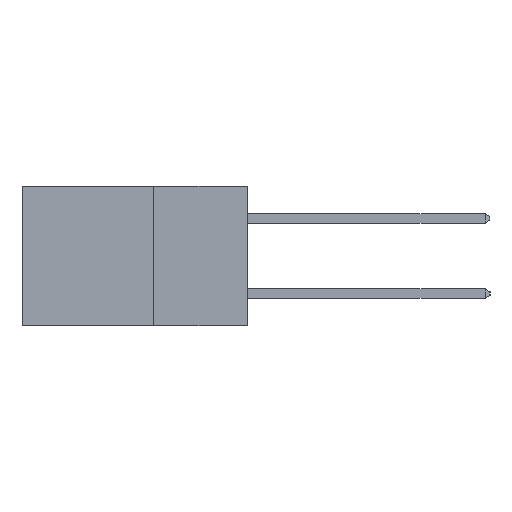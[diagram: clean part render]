
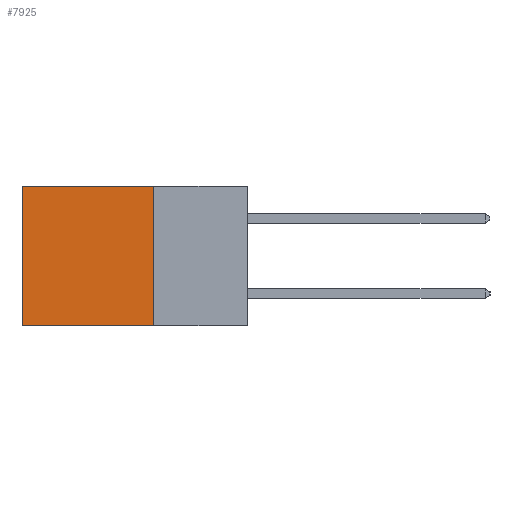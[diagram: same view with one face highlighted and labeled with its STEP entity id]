
A CAD part, left-side view. The second image highlights one B-rep face of the part: STEP entity #7925.
In plain terms, the highlighted planar face has unit normal (-1, 0, 0).
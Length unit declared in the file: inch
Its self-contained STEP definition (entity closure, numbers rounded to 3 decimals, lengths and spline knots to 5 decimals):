
#203 = LINE ( 'NONE', #7552, #11083 ) ;
#416 = DIRECTION ( 'NONE',  ( 0., 0., -1. ) ) ;
#539 = CARTESIAN_POINT ( 'NONE',  ( 0.2615, 0.6, -0.37 ) ) ;
#847 = CARTESIAN_POINT ( 'NONE',  ( 0.2615, 0.6, 0. ) ) ;
#979 = CARTESIAN_POINT ( 'NONE',  ( 0.2615, 0.25, -0.37 ) ) ;
#1391 = ORIENTED_EDGE ( 'NONE', *, *, #9194, .F. ) ;
#1603 = DIRECTION ( 'NONE',  ( 0., 1., 0. ) ) ;
#1889 = DIRECTION ( 'NONE',  ( 1., 0., 0. ) ) ;
#2540 = EDGE_CURVE ( 'NONE', #7242, #8028, #10541, .T. ) ;
#2684 = VECTOR ( 'NONE', #7913, 39.37008 ) ;
#3833 = PLANE ( 'NONE',  #10308 ) ;
#5373 = CARTESIAN_POINT ( 'NONE',  ( 0.2615, 0.25, -0.37 ) ) ;
#5421 = CARTESIAN_POINT ( 'NONE',  ( 0.2615, 0.25, -0.37 ) ) ;
#5601 = VERTEX_POINT ( 'NONE', #5373 ) ;
#5627 = EDGE_CURVE ( 'NONE', #7146, #5601, #10991, .T. ) ;
#6602 = EDGE_LOOP ( 'NONE', ( #6776, #1391, #6907, #6700 ) ) ;
#6700 = ORIENTED_EDGE ( 'NONE', *, *, #11740, .T. ) ;
#6776 = ORIENTED_EDGE ( 'NONE', *, *, #2540, .T. ) ;
#6907 = ORIENTED_EDGE ( 'NONE', *, *, #5627, .F. ) ;
#7146 = VERTEX_POINT ( 'NONE', #8659 ) ;
#7242 = VERTEX_POINT ( 'NONE', #847 ) ;
#7552 = CARTESIAN_POINT ( 'NONE',  ( 0.2615, 0.25, 0. ) ) ;
#7913 = DIRECTION ( 'NONE',  ( 0., 1., 0. ) ) ;
#7925 = ADVANCED_FACE ( 'NONE', ( #9550 ), #3833, .F. ) ;
#8028 = VERTEX_POINT ( 'NONE', #10957 ) ;
#8659 = CARTESIAN_POINT ( 'NONE',  ( 0.2615, 0.25, 0. ) ) ;
#8826 = DIRECTION ( 'NONE',  ( 0., 0., -1. ) ) ;
#9194 = EDGE_CURVE ( 'NONE', #5601, #8028, #10310, .T. ) ;
#9550 = FACE_OUTER_BOUND ( 'NONE', #6602, .T. ) ;
#10308 = AXIS2_PLACEMENT_3D ( 'NONE', #10788, #1889, #8826 ) ;
#10310 = LINE ( 'NONE', #979, #2684 ) ;
#10541 = LINE ( 'NONE', #539, #10845 ) ;
#10692 = VECTOR ( 'NONE', #416, 39.37008 ) ;
#10788 = CARTESIAN_POINT ( 'NONE',  ( 0.2615, 0.25, -0.37 ) ) ;
#10845 = VECTOR ( 'NONE', #12333, 39.37008 ) ;
#10957 = CARTESIAN_POINT ( 'NONE',  ( 0.2615, 0.6, -0.37 ) ) ;
#10991 = LINE ( 'NONE', #5421, #10692 ) ;
#11083 = VECTOR ( 'NONE', #1603, 39.37008 ) ;
#11740 = EDGE_CURVE ( 'NONE', #7146, #7242, #203, .T. ) ;
#12333 = DIRECTION ( 'NONE',  ( 0., 0., -1. ) ) ;
